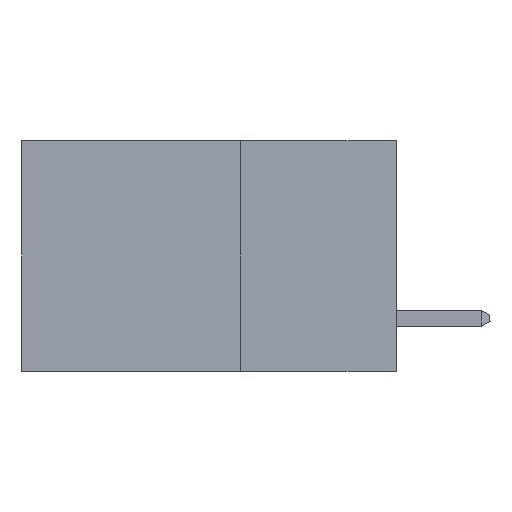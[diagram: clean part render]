
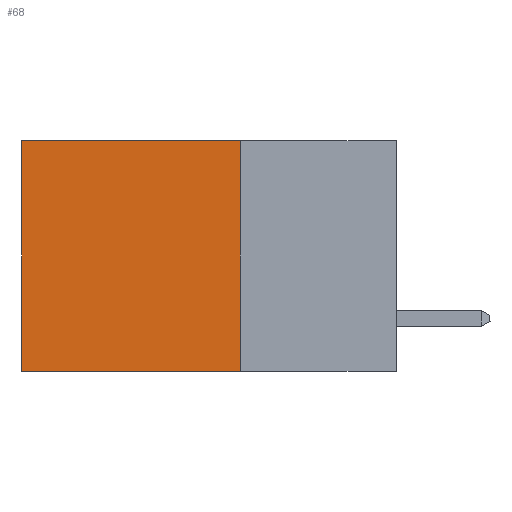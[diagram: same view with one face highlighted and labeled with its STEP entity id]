
A CAD part, left-side view. The second image highlights one B-rep face of the part: STEP entity #68.
In plain terms, the highlighted planar face has unit normal (-1, 0, 0).
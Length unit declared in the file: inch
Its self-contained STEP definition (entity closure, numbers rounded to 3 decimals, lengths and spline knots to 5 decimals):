
#25 = AXIS2_PLACEMENT_3D ( 'NONE', #9077, #2781, #10099 ) ;
#35 = LINE ( 'NONE', #2963, #2240 ) ;
#68 = ADVANCED_FACE ( 'NONE', ( #1712 ), #3831, .F. ) ;
#164 = LINE ( 'NONE', #4532, #10917 ) ;
#220 = EDGE_CURVE ( 'NONE', #4279, #6802, #1028, .T. ) ;
#487 = DIRECTION ( 'NONE',  ( 0., 1., 0. ) ) ;
#702 = CARTESIAN_POINT ( 'NONE',  ( 0.298, 0.25, 0. ) ) ;
#1028 = LINE ( 'NONE', #4201, #10002 ) ;
#1158 = CARTESIAN_POINT ( 'NONE',  ( 0.298, 0.25, -0.37 ) ) ;
#1214 = EDGE_CURVE ( 'NONE', #4279, #2208, #35, .T. ) ;
#1254 = DIRECTION ( 'NONE',  ( 0., 0., -1. ) ) ;
#1379 = EDGE_LOOP ( 'NONE', ( #9804, #8857, #2631, #2305 ) ) ;
#1418 = EDGE_CURVE ( 'NONE', #6802, #1546, #164, .T. ) ;
#1546 = VERTEX_POINT ( 'NONE', #9561 ) ;
#1712 = FACE_OUTER_BOUND ( 'NONE', #1379, .T. ) ;
#2208 = VERTEX_POINT ( 'NONE', #1158 ) ;
#2240 = VECTOR ( 'NONE', #1254, 39.37008 ) ;
#2305 = ORIENTED_EDGE ( 'NONE', *, *, #220, .T. ) ;
#2631 = ORIENTED_EDGE ( 'NONE', *, *, #1214, .F. ) ;
#2712 = DIRECTION ( 'NONE',  ( 0., 0., -1. ) ) ;
#2781 = DIRECTION ( 'NONE',  ( 1., 0., 0. ) ) ;
#2963 = CARTESIAN_POINT ( 'NONE',  ( 0.298, 0.25, 0. ) ) ;
#2964 = DIRECTION ( 'NONE',  ( 0., 1., 0. ) ) ;
#3831 = PLANE ( 'NONE',  #25 ) ;
#4201 = CARTESIAN_POINT ( 'NONE',  ( 0.298, 0.25, 0. ) ) ;
#4279 = VERTEX_POINT ( 'NONE', #702 ) ;
#4532 = CARTESIAN_POINT ( 'NONE',  ( 0.298, 0.6, 0. ) ) ;
#4641 = EDGE_CURVE ( 'NONE', #2208, #1546, #11390, .T. ) ;
#5924 = CARTESIAN_POINT ( 'NONE',  ( 0.298, 0.6, 0. ) ) ;
#6802 = VERTEX_POINT ( 'NONE', #5924 ) ;
#8351 = CARTESIAN_POINT ( 'NONE',  ( 0.298, 0.25, -0.37 ) ) ;
#8780 = VECTOR ( 'NONE', #2964, 39.37008 ) ;
#8857 = ORIENTED_EDGE ( 'NONE', *, *, #4641, .F. ) ;
#9077 = CARTESIAN_POINT ( 'NONE',  ( 0.298, 0.25, 0. ) ) ;
#9561 = CARTESIAN_POINT ( 'NONE',  ( 0.298, 0.6, -0.37 ) ) ;
#9804 = ORIENTED_EDGE ( 'NONE', *, *, #1418, .T. ) ;
#10002 = VECTOR ( 'NONE', #487, 39.37008 ) ;
#10099 = DIRECTION ( 'NONE',  ( 0., 0., -1. ) ) ;
#10917 = VECTOR ( 'NONE', #2712, 39.37008 ) ;
#11390 = LINE ( 'NONE', #8351, #8780 ) ;
